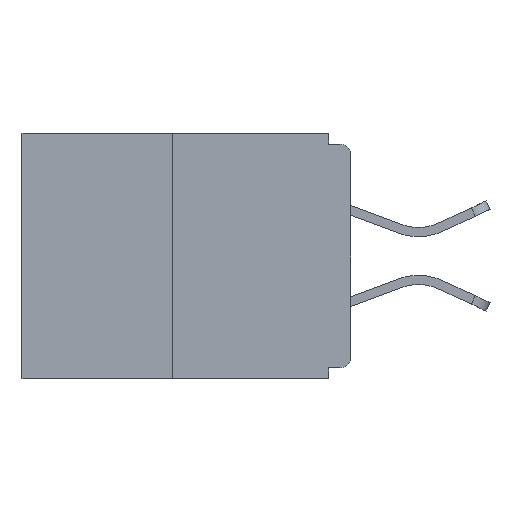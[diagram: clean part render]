
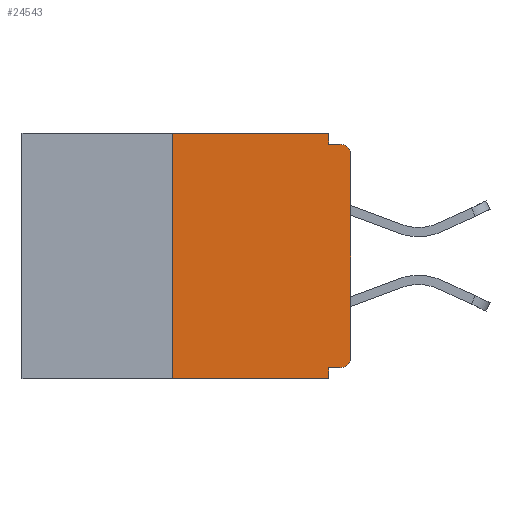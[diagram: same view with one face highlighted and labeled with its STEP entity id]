
A CAD part, left-side view. The second image highlights one B-rep face of the part: STEP entity #24543.
In plain terms, the highlighted planar face has unit normal (-1, 0, 0).
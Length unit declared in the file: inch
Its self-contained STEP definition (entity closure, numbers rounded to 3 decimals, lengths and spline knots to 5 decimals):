
#31 = VERTEX_POINT ( 'NONE', #21076 ) ;
#264 = LINE ( 'NONE', #2187, #16422 ) ;
#306 = VERTEX_POINT ( 'NONE', #2374 ) ;
#533 = CARTESIAN_POINT ( 'NONE',  ( 0., 0.031, -0.343 ) ) ;
#555 = EDGE_CURVE ( 'NONE', #14716, #7148, #1688, .T. ) ;
#601 = VERTEX_POINT ( 'NONE', #14632 ) ;
#1330 = ORIENTED_EDGE ( 'NONE', *, *, #14884, .T. ) ;
#1688 = LINE ( 'NONE', #16730, #13677 ) ;
#2187 = CARTESIAN_POINT ( 'NONE',  ( 0., 0.25, 0. ) ) ;
#2233 = ORIENTED_EDGE ( 'NONE', *, *, #18087, .F. ) ;
#2374 = CARTESIAN_POINT ( 'NONE',  ( 0., 0.25, -0.343 ) ) ;
#2466 = ORIENTED_EDGE ( 'NONE', *, *, #3161, .F. ) ;
#2899 = AXIS2_PLACEMENT_3D ( 'NONE', #14779, #7230, #9064 ) ;
#3161 = EDGE_CURVE ( 'NONE', #7148, #17890, #9038, .T. ) ;
#3335 = CARTESIAN_POINT ( 'NONE',  ( 0., 0., 0. ) ) ;
#4267 = FACE_OUTER_BOUND ( 'NONE', #18213, .T. ) ;
#4340 = VERTEX_POINT ( 'NONE', #533 ) ;
#4610 = ORIENTED_EDGE ( 'NONE', *, *, #5682, .F. ) ;
#5682 = EDGE_CURVE ( 'NONE', #306, #31, #264, .T. ) ;
#5782 = CARTESIAN_POINT ( 'NONE',  ( 0., 0., -0.328 ) ) ;
#6121 = DIRECTION ( 'NONE',  ( 0., 0., 1. ) ) ;
#6280 = AXIS2_PLACEMENT_3D ( 'NONE', #24602, #13499, #7634 ) ;
#6464 = EDGE_CURVE ( 'NONE', #24355, #7556, #11620, .T. ) ;
#6495 = VECTOR ( 'NONE', #23171, 39.37008 ) ;
#6804 = CARTESIAN_POINT ( 'NONE',  ( 0., 0.46, 0. ) ) ;
#7075 = DIRECTION ( 'NONE',  ( -1., 0., 0. ) ) ;
#7148 = VERTEX_POINT ( 'NONE', #20276 ) ;
#7230 = DIRECTION ( 'NONE',  ( -1., 0., 0. ) ) ;
#7556 = VERTEX_POINT ( 'NONE', #16254 ) ;
#7634 = DIRECTION ( 'NONE',  ( 0., 0., -1. ) ) ;
#8578 = LINE ( 'NONE', #11463, #6495 ) ;
#8924 = DIRECTION ( 'NONE',  ( 0., 0., -1. ) ) ;
#9038 = LINE ( 'NONE', #23265, #23722 ) ;
#9064 = DIRECTION ( 'NONE',  ( 0., 0., -1. ) ) ;
#9312 = LINE ( 'NONE', #5782, #23980 ) ;
#9762 = VERTEX_POINT ( 'NONE', #16463 ) ;
#10169 = EDGE_CURVE ( 'NONE', #306, #4340, #15680, .T. ) ;
#10545 = ORIENTED_EDGE ( 'NONE', *, *, #10169, .T. ) ;
#10859 = AXIS2_PLACEMENT_3D ( 'NONE', #16464, #7075, #8924 ) ;
#11410 = PLANE ( 'NONE',  #6280 ) ;
#11463 = CARTESIAN_POINT ( 'NONE',  ( 0., 0.031, -0.343 ) ) ;
#11620 = LINE ( 'NONE', #3335, #23586 ) ;
#12057 = VECTOR ( 'NONE', #23395, 39.37008 ) ;
#12523 = ORIENTED_EDGE ( 'NONE', *, *, #6464, .T. ) ;
#12525 = ORIENTED_EDGE ( 'NONE', *, *, #15467, .F. ) ;
#12782 = LINE ( 'NONE', #6804, #19982 ) ;
#12841 = DIRECTION ( 'NONE',  ( 0., -1., 0. ) ) ;
#13099 = CARTESIAN_POINT ( 'NONE',  ( 0., 0., -0.313 ) ) ;
#13499 = DIRECTION ( 'NONE',  ( 1., 0., 0. ) ) ;
#13677 = VECTOR ( 'NONE', #16479, 39.37008 ) ;
#13770 = CARTESIAN_POINT ( 'NONE',  ( 0., 0.46, -0.343 ) ) ;
#13920 = CARTESIAN_POINT ( 'NONE',  ( 0., 0.031, 0. ) ) ;
#14089 = ORIENTED_EDGE ( 'NONE', *, *, #24571, .F. ) ;
#14632 = CARTESIAN_POINT ( 'NONE',  ( 0., 0.031, -0.328 ) ) ;
#14716 = VERTEX_POINT ( 'NONE', #13920 ) ;
#14779 = CARTESIAN_POINT ( 'NONE',  ( 0., 0.015, -0.313 ) ) ;
#14884 = EDGE_CURVE ( 'NONE', #9762, #24355, #19721, .T. ) ;
#15467 = EDGE_CURVE ( 'NONE', #31, #14716, #12782, .T. ) ;
#15680 = LINE ( 'NONE', #13770, #12057 ) ;
#16254 = CARTESIAN_POINT ( 'NONE',  ( 0., 0., -0.03 ) ) ;
#16259 = CARTESIAN_POINT ( 'NONE',  ( 0., 0.015, -0.015 ) ) ;
#16422 = VECTOR ( 'NONE', #6121, 39.37008 ) ;
#16463 = CARTESIAN_POINT ( 'NONE',  ( 0., 0.015, -0.328 ) ) ;
#16464 = CARTESIAN_POINT ( 'NONE',  ( 0., 0.015, -0.03 ) ) ;
#16479 = DIRECTION ( 'NONE',  ( 0., 0., -1. ) ) ;
#16730 = CARTESIAN_POINT ( 'NONE',  ( 0., 0.031, 0. ) ) ;
#16901 = DIRECTION ( 'NONE',  ( 0., 0., 1. ) ) ;
#17890 = VERTEX_POINT ( 'NONE', #16259 ) ;
#18060 = ORIENTED_EDGE ( 'NONE', *, *, #555, .F. ) ;
#18087 = EDGE_CURVE ( 'NONE', #601, #4340, #8578, .T. ) ;
#18213 = EDGE_LOOP ( 'NONE', ( #12525, #4610, #10545, #2233, #14089, #1330, #12523, #19763, #2466, #18060 ) ) ;
#19188 = DIRECTION ( 'NONE',  ( 0., 1., 0. ) ) ;
#19721 = CIRCLE ( 'NONE', #2899, 0.015 ) ;
#19763 = ORIENTED_EDGE ( 'NONE', *, *, #20914, .T. ) ;
#19982 = VECTOR ( 'NONE', #12841, 39.37008 ) ;
#20276 = CARTESIAN_POINT ( 'NONE',  ( 0., 0.031, -0.015 ) ) ;
#20914 = EDGE_CURVE ( 'NONE', #7556, #17890, #23486, .T. ) ;
#21076 = CARTESIAN_POINT ( 'NONE',  ( 0., 0.25, 0. ) ) ;
#21175 = DIRECTION ( 'NONE',  ( 0., -1., 0. ) ) ;
#23171 = DIRECTION ( 'NONE',  ( 0., 0., -1. ) ) ;
#23265 = CARTESIAN_POINT ( 'NONE',  ( 0., 0., -0.015 ) ) ;
#23395 = DIRECTION ( 'NONE',  ( 0., -1., 0. ) ) ;
#23486 = CIRCLE ( 'NONE', #10859, 0.015 ) ;
#23586 = VECTOR ( 'NONE', #16901, 39.37008 ) ;
#23722 = VECTOR ( 'NONE', #21175, 39.37008 ) ;
#23980 = VECTOR ( 'NONE', #19188, 39.37008 ) ;
#24355 = VERTEX_POINT ( 'NONE', #13099 ) ;
#24543 = ADVANCED_FACE ( 'NONE', ( #4267 ), #11410, .F. ) ;
#24571 = EDGE_CURVE ( 'NONE', #9762, #601, #9312, .T. ) ;
#24602 = CARTESIAN_POINT ( 'NONE',  ( 0., 0.46, 0. ) ) ;
